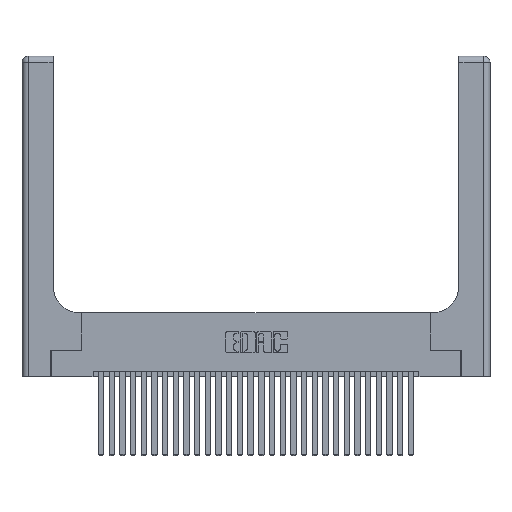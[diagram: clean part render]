
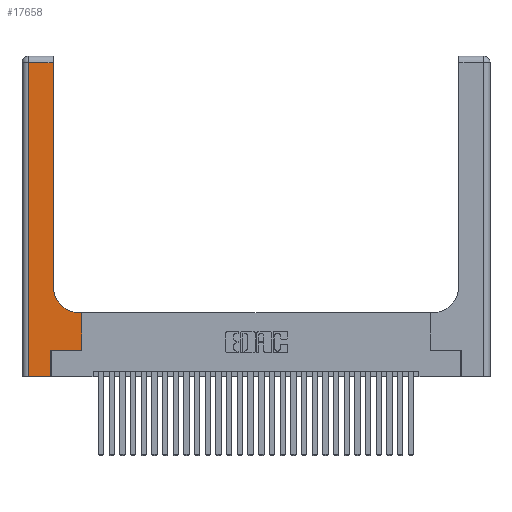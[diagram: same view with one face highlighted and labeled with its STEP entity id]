
A CAD part, top view. The second image highlights one B-rep face of the part: STEP entity #17658.
In plain terms, the highlighted planar face has unit normal (0, 0, 1).
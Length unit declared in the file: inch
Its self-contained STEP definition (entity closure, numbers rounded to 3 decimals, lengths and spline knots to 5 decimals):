
#41 = LINE ( 'NONE', #10638, #24859 ) ;
#212 = ORIENTED_EDGE ( 'NONE', *, *, #10858, .T. ) ;
#294 = CARTESIAN_POINT ( 'NONE',  ( 0., 0., 0.37 ) ) ;
#1138 = ORIENTED_EDGE ( 'NONE', *, *, #4204, .T. ) ;
#1143 = VECTOR ( 'NONE', #9571, 39.37008 ) ;
#1165 = ORIENTED_EDGE ( 'NONE', *, *, #7935, .T. ) ;
#1613 = CARTESIAN_POINT ( 'NONE',  ( 0.5585, 0.6, 0.37 ) ) ;
#2016 = LINE ( 'NONE', #4521, #22085 ) ;
#2305 = LINE ( 'NONE', #24406, #19065 ) ;
#2338 = VECTOR ( 'NONE', #17398, 39.37008 ) ;
#2474 = CARTESIAN_POINT ( 'NONE',  ( 0.06, 3., 0.37 ) ) ;
#3643 = VECTOR ( 'NONE', #23691, 39.37008 ) ;
#3792 = VECTOR ( 'NONE', #15180, 39.37008 ) ;
#3904 = VERTEX_POINT ( 'NONE', #29688 ) ;
#4204 = EDGE_CURVE ( 'NONE', #14841, #13085, #10913, .T. ) ;
#4521 = CARTESIAN_POINT ( 'NONE',  ( 0.269, 0.25, 0.37 ) ) ;
#4524 = LINE ( 'NONE', #29228, #3792 ) ;
#6412 = EDGE_CURVE ( 'NONE', #17755, #7226, #2016, .T. ) ;
#7226 = VERTEX_POINT ( 'NONE', #19828 ) ;
#7765 = LINE ( 'NONE', #7925, #2338 ) ;
#7770 = EDGE_CURVE ( 'NONE', #25697, #17755, #2305, .T. ) ;
#7925 = CARTESIAN_POINT ( 'NONE',  ( 0.5585, 0.25, 0.37 ) ) ;
#7935 = EDGE_CURVE ( 'NONE', #8525, #3904, #10309, .T. ) ;
#8525 = VERTEX_POINT ( 'NONE', #1613 ) ;
#8792 = ORIENTED_EDGE ( 'NONE', *, *, #22112, .T. ) ;
#8952 = CARTESIAN_POINT ( 'NONE',  ( 0.269, 0., 0.37 ) ) ;
#9571 = DIRECTION ( 'NONE',  ( 1., 0., 0. ) ) ;
#10039 = PLANE ( 'NONE',  #13798 ) ;
#10309 = LINE ( 'NONE', #18602, #14687 ) ;
#10360 = CARTESIAN_POINT ( 'NONE',  ( 0.06, 0., 0.37 ) ) ;
#10398 = DIRECTION ( 'NONE',  ( 0., 1., 0. ) ) ;
#10399 = DIRECTION ( 'NONE',  ( 1., 0., 0. ) ) ;
#10638 = CARTESIAN_POINT ( 'NONE',  ( 0., 2.94, 0.37 ) ) ;
#10858 = EDGE_CURVE ( 'NONE', #13446, #14841, #41, .T. ) ;
#10913 = LINE ( 'NONE', #2474, #3643 ) ;
#12417 = DIRECTION ( 'NONE',  ( 0., 0., -1. ) ) ;
#12750 = ORIENTED_EDGE ( 'NONE', *, *, #6412, .T. ) ;
#13085 = VERTEX_POINT ( 'NONE', #10360 ) ;
#13446 = VERTEX_POINT ( 'NONE', #25064 ) ;
#13798 = AXIS2_PLACEMENT_3D ( 'NONE', #14654, #12417, #16871 ) ;
#14654 = CARTESIAN_POINT ( 'NONE',  ( 0., 3., 0.37 ) ) ;
#14687 = VECTOR ( 'NONE', #30092, 39.37008 ) ;
#14841 = VERTEX_POINT ( 'NONE', #18992 ) ;
#15180 = DIRECTION ( 'NONE',  ( 0., 1., 0. ) ) ;
#15405 = DIRECTION ( 'NONE',  ( 0., 0., -1. ) ) ;
#15500 = CIRCLE ( 'NONE', #29347, 0.25 ) ;
#16774 = CARTESIAN_POINT ( 'NONE',  ( 0.269, 0.25, 0.37 ) ) ;
#16871 = DIRECTION ( 'NONE',  ( -1., 0., 0. ) ) ;
#17188 = ORIENTED_EDGE ( 'NONE', *, *, #27352, .T. ) ;
#17260 = EDGE_CURVE ( 'NONE', #23046, #13446, #4524, .T. ) ;
#17398 = DIRECTION ( 'NONE',  ( 0., 1., 0. ) ) ;
#17658 = ADVANCED_FACE ( 'NONE', ( #24930 ), #10039, .F. ) ;
#17755 = VERTEX_POINT ( 'NONE', #16774 ) ;
#17927 = LINE ( 'NONE', #294, #1143 ) ;
#18602 = CARTESIAN_POINT ( 'NONE',  ( 0.2915, 0.6, 0.37 ) ) ;
#18992 = CARTESIAN_POINT ( 'NONE',  ( 0.06, 2.94, 0.37 ) ) ;
#19065 = VECTOR ( 'NONE', #10398, 39.37008 ) ;
#19828 = CARTESIAN_POINT ( 'NONE',  ( 0.5585, 0.25, 0.37 ) ) ;
#21713 = ORIENTED_EDGE ( 'NONE', *, *, #26724, .T. ) ;
#22085 = VECTOR ( 'NONE', #22928, 39.37008 ) ;
#22112 = EDGE_CURVE ( 'NONE', #13085, #25697, #17927, .T. ) ;
#22928 = DIRECTION ( 'NONE',  ( 1., 0., 0. ) ) ;
#23046 = VERTEX_POINT ( 'NONE', #28790 ) ;
#23691 = DIRECTION ( 'NONE',  ( 0., -1., 0. ) ) ;
#24406 = CARTESIAN_POINT ( 'NONE',  ( 0.269, 0., 0.37 ) ) ;
#24664 = ORIENTED_EDGE ( 'NONE', *, *, #7770, .T. ) ;
#24859 = VECTOR ( 'NONE', #27260, 39.37008 ) ;
#24930 = FACE_OUTER_BOUND ( 'NONE', #27666, .T. ) ;
#25064 = CARTESIAN_POINT ( 'NONE',  ( 0.2915, 2.94, 0.37 ) ) ;
#25697 = VERTEX_POINT ( 'NONE', #8952 ) ;
#26724 = EDGE_CURVE ( 'NONE', #3904, #23046, #15500, .T. ) ;
#27260 = DIRECTION ( 'NONE',  ( -1., 0., 0. ) ) ;
#27352 = EDGE_CURVE ( 'NONE', #7226, #8525, #7765, .T. ) ;
#27666 = EDGE_LOOP ( 'NONE', ( #28965, #212, #1138, #8792, #24664, #12750, #17188, #1165, #21713 ) ) ;
#28790 = CARTESIAN_POINT ( 'NONE',  ( 0.2915, 0.85, 0.37 ) ) ;
#28965 = ORIENTED_EDGE ( 'NONE', *, *, #17260, .T. ) ;
#29228 = CARTESIAN_POINT ( 'NONE',  ( 0.2915, 3., 0.37 ) ) ;
#29347 = AXIS2_PLACEMENT_3D ( 'NONE', #29359, #15405, #10399 ) ;
#29359 = CARTESIAN_POINT ( 'NONE',  ( 0.5415, 0.85, 0.37 ) ) ;
#29688 = CARTESIAN_POINT ( 'NONE',  ( 0.5415, 0.6, 0.37 ) ) ;
#30092 = DIRECTION ( 'NONE',  ( -1., 0., 0. ) ) ;
